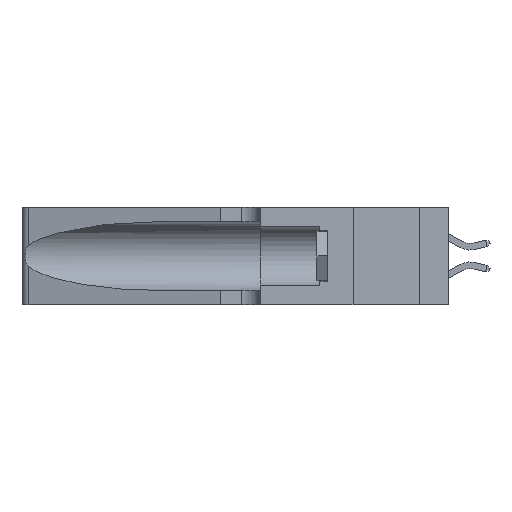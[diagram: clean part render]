
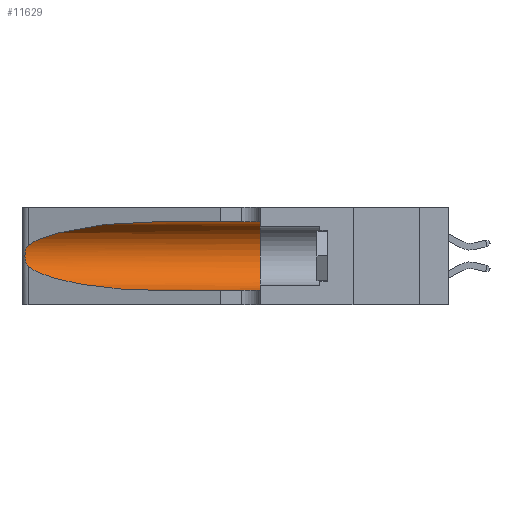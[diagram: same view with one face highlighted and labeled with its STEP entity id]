
A CAD part, left-side view. The second image highlights one B-rep face of the part: STEP entity #11629.
In plain terms, the highlighted cylindrical face has radius 3.308 mm (diameter 6.617 mm), a partial arc.
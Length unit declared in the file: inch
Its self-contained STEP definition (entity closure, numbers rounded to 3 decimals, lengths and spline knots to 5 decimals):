
#113 = CARTESIAN_POINT ( 'NONE',  ( 0.2373, 1.15595, 0.28018 ) ) ;
#299 = B_SPLINE_CURVE_WITH_KNOTS ( 'NONE', 3,
 ( #16056, #36516, #29770, #9215, #33203, #12710, #36668, #16198, #40044, #19663, #43468, #23113, #2218, #26544 ),
 .UNSPECIFIED., .F., .F.,
 ( 4, 2, 2, 2, 2, 2, 4 ),
 ( 0., 0.00027, 0.00053, 0.00107, 0.0016, 0.00187, 0.00214 ),
 .UNSPECIFIED. ) ;
#1706 = EDGE_CURVE ( 'NONE', #31291, #17165, #37338, .T. ) ;
#1830 = ORIENTED_EDGE ( 'NONE', *, *, #43618, .T. ) ;
#2218 = CARTESIAN_POINT ( 'NONE',  ( 0.25555, 1.22993, 0.14849 ) ) ;
#3292 = CARTESIAN_POINT ( 'NONE',  ( 0.1305, 0.72297, 0.31525 ) ) ;
#3651 = CARTESIAN_POINT ( 'NONE',  ( 0.25487, 1.22718, 0.22369 ) ) ;
#3998 = VERTEX_POINT ( 'NONE', #39240 ) ;
#4169 = CARTESIAN_POINT ( 'NONE',  ( 0.25487, 1.22718, 0.14631 ) ) ;
#4426 = EDGE_CURVE ( 'NONE', #37798, #12574, #19939, .T. ) ;
#4486 = DIRECTION ( 'NONE',  ( 0., -1., 0. ) ) ;
#7064 = CARTESIAN_POINT ( 'NONE',  ( 0.18966, 0.96281, 0.31525 ) ) ;
#7729 = CARTESIAN_POINT ( 'NONE',  ( 0.18966, 0.96281, 0.05475 ) ) ;
#9215 = CARTESIAN_POINT ( 'NONE',  ( 0.25787, 1.23484, 0.2124 ) ) ;
#11629 = ADVANCED_FACE ( 'NONE', ( #15546 ), #23588, .F. ) ;
#12574 = VERTEX_POINT ( 'NONE', #27871 ) ;
#12710 = CARTESIAN_POINT ( 'NONE',  ( 0.26018, 1.23835, 0.19895 ) ) ;
#14626 = CARTESIAN_POINT ( 'NONE',  ( 0.2373, 1.15595, 0.08982 ) ) ;
#15392 = VERTEX_POINT ( 'NONE', #19016 ) ;
#15546 = FACE_OUTER_BOUND ( 'NONE', #21509, .T. ) ;
#16056 = CARTESIAN_POINT ( 'NONE',  ( 0.25487, 1.22718, 0.22369 ) ) ;
#16198 = CARTESIAN_POINT ( 'NONE',  ( 0.26075, 1.23896, 0.178 ) ) ;
#17037 = DIRECTION ( 'NONE',  ( 0., 1., 0. ) ) ;
#17165 = VERTEX_POINT ( 'NONE', #31963 ) ;
#19016 = CARTESIAN_POINT ( 'NONE',  ( 0.25487, 1.22718, 0.14631 ) ) ;
#19663 = CARTESIAN_POINT ( 'NONE',  ( 0.25856, 1.23593, 0.16098 ) ) ;
#19939 =( BOUNDED_CURVE ( )  B_SPLINE_CURVE ( 3, ( #41415, #7064, #113, #3651 ),
 .UNSPECIFIED., .F., .F. ) 
 B_SPLINE_CURVE_WITH_KNOTS ( ( 4, 4 ),
 ( 1.5708, 2.84003 ),
 .UNSPECIFIED. ) 
 CURVE ( )  GEOMETRIC_REPRESENTATION_ITEM ( )  RATIONAL_B_SPLINE_CURVE ( ( 1., 0.87, 0.87, 1. ) ) 
 REPRESENTATION_ITEM ( '' )  );
#21144 = DIRECTION ( 'NONE',  ( 0., -1., 0. ) ) ;
#21509 = EDGE_LOOP ( 'NONE', ( #40623, #22087, #1830, #33019, #33464, #21775 ) ) ;
#21775 = ORIENTED_EDGE ( 'NONE', *, *, #25327, .F. ) ;
#21848 = CARTESIAN_POINT ( 'NONE',  ( 0.1305, 1.61858, 0.31525 ) ) ;
#22087 = ORIENTED_EDGE ( 'NONE', *, *, #34749, .T. ) ;
#23113 = CARTESIAN_POINT ( 'NONE',  ( 0.25639, 1.23186, 0.15144 ) ) ;
#23588 = CYLINDRICAL_SURFACE ( 'NONE', #41805, 0.13025 ) ;
#25181 = AXIS2_PLACEMENT_3D ( 'NONE', #37483, #17037, #40865 ) ;
#25327 = EDGE_CURVE ( 'NONE', #37798, #3998, #42343, .T. ) ;
#26544 = CARTESIAN_POINT ( 'NONE',  ( 0.25487, 1.22718, 0.14631 ) ) ;
#26635 = CARTESIAN_POINT ( 'NONE',  ( 0.1305, 1.61858, 0.185 ) ) ;
#27871 = CARTESIAN_POINT ( 'NONE',  ( 0.25487, 1.22718, 0.22369 ) ) ;
#29770 = CARTESIAN_POINT ( 'NONE',  ( 0.25639, 1.23184, 0.21858 ) ) ;
#31291 = VERTEX_POINT ( 'NONE', #38112 ) ;
#31776 = CARTESIAN_POINT ( 'NONE',  ( 0.1305, 0.72297, 0.05475 ) ) ;
#31963 = CARTESIAN_POINT ( 'NONE',  ( 0.1305, 0.35, 0.05475 ) ) ;
#33019 = ORIENTED_EDGE ( 'NONE', *, *, #1706, .T. ) ;
#33203 = CARTESIAN_POINT ( 'NONE',  ( 0.25854, 1.2359, 0.20912 ) ) ;
#33295 = VECTOR ( 'NONE', #4486, 39.37008 ) ;
#33464 = ORIENTED_EDGE ( 'NONE', *, *, #35587, .F. ) ;
#34749 = EDGE_CURVE ( 'NONE', #12574, #15392, #299, .T. ) ;
#35587 = EDGE_CURVE ( 'NONE', #3998, #17165, #36547, .T. ) ;
#36267 = VECTOR ( 'NONE', #21144, 39.37008 ) ;
#36516 = CARTESIAN_POINT ( 'NONE',  ( 0.25555, 1.22994, 0.2215 ) ) ;
#36547 = CIRCLE ( 'NONE', #25181, 0.13025 ) ;
#36668 = CARTESIAN_POINT ( 'NONE',  ( 0.26075, 1.23896, 0.19203 ) ) ;
#37338 = LINE ( 'NONE', #38272, #36267 ) ;
#37483 = CARTESIAN_POINT ( 'NONE',  ( 0.1305, 0.35, 0.185 ) ) ;
#37798 = VERTEX_POINT ( 'NONE', #3292 ) ;
#38112 = CARTESIAN_POINT ( 'NONE',  ( 0.1305, 0.72297, 0.05475 ) ) ;
#38272 = CARTESIAN_POINT ( 'NONE',  ( 0.1305, 1.61858, 0.05475 ) ) ;
#39240 = CARTESIAN_POINT ( 'NONE',  ( 0.1305, 0.35, 0.31525 ) ) ;
#40044 = CARTESIAN_POINT ( 'NONE',  ( 0.26017, 1.23833, 0.17102 ) ) ;
#40292 = DIRECTION ( 'NONE',  ( 0., -1., 0. ) ) ;
#40623 = ORIENTED_EDGE ( 'NONE', *, *, #4426, .T. ) ;
#40865 = DIRECTION ( 'NONE',  ( 0., 0., 1. ) ) ;
#41415 = CARTESIAN_POINT ( 'NONE',  ( 0.1305, 0.72297, 0.31525 ) ) ;
#41741 =( BOUNDED_CURVE ( )  B_SPLINE_CURVE ( 3, ( #4169, #14626, #7729, #31776 ),
 .UNSPECIFIED., .F., .F. ) 
 B_SPLINE_CURVE_WITH_KNOTS ( ( 4, 4 ),
 ( 3.44316, 4.71239 ),
 .UNSPECIFIED. ) 
 CURVE ( )  GEOMETRIC_REPRESENTATION_ITEM ( )  RATIONAL_B_SPLINE_CURVE ( ( 1., 0.87, 0.87, 1. ) ) 
 REPRESENTATION_ITEM ( '' )  );
#41805 = AXIS2_PLACEMENT_3D ( 'NONE', #26635, #40292, #43694 ) ;
#42343 = LINE ( 'NONE', #21848, #33295 ) ;
#43468 = CARTESIAN_POINT ( 'NONE',  ( 0.25789, 1.23486, 0.15765 ) ) ;
#43618 = EDGE_CURVE ( 'NONE', #15392, #31291, #41741, .T. ) ;
#43694 = DIRECTION ( 'NONE',  ( 0., 0., -1. ) ) ;
